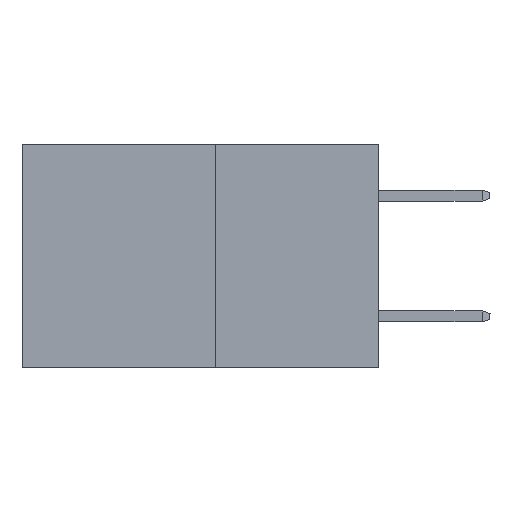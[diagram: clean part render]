
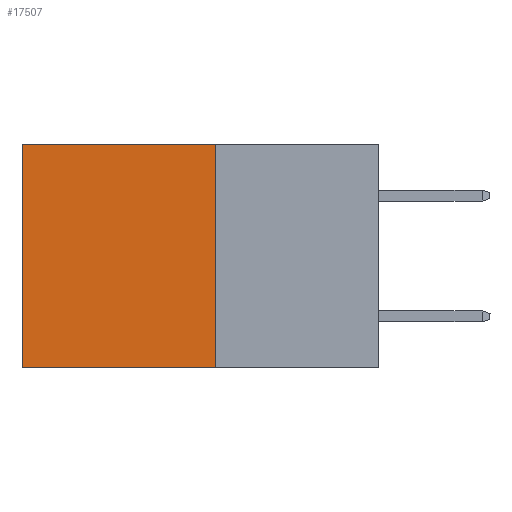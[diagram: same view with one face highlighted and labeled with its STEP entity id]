
A CAD part, left-side view. The second image highlights one B-rep face of the part: STEP entity #17507.
In plain terms, the highlighted planar face has unit normal (-1, 0, 0).
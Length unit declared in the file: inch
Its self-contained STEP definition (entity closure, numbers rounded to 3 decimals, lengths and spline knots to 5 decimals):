
#2429 = LINE ( 'NONE', #11692, #23320 ) ;
#3173 = EDGE_CURVE ( 'NONE', #24598, #13767, #14468, .T. ) ;
#4487 = VERTEX_POINT ( 'NONE', #9803 ) ;
#5060 = AXIS2_PLACEMENT_3D ( 'NONE', #27791, #23147, #8658 ) ;
#5334 = VERTEX_POINT ( 'NONE', #18171 ) ;
#6518 = EDGE_CURVE ( 'NONE', #4487, #5334, #2429, .T. ) ;
#7729 = CARTESIAN_POINT ( 'NONE',  ( 0.277, 0.27, -0.37 ) ) ;
#7737 = ORIENTED_EDGE ( 'NONE', *, *, #30972, .T. ) ;
#8658 = DIRECTION ( 'NONE',  ( 0., 0., -1. ) ) ;
#9319 = ORIENTED_EDGE ( 'NONE', *, *, #6518, .F. ) ;
#9803 = CARTESIAN_POINT ( 'NONE',  ( 0.277, 0.27, 0. ) ) ;
#10033 = FACE_OUTER_BOUND ( 'NONE', #12691, .T. ) ;
#10631 = EDGE_CURVE ( 'NONE', #5334, #13767, #21751, .T. ) ;
#10875 = VECTOR ( 'NONE', #20563, 39.37008 ) ;
#11692 = CARTESIAN_POINT ( 'NONE',  ( 0.277, 0.27, -0.37 ) ) ;
#12691 = EDGE_LOOP ( 'NONE', ( #21202, #16113, #9319, #7737 ) ) ;
#13726 = VECTOR ( 'NONE', #25982, 39.37008 ) ;
#13767 = VERTEX_POINT ( 'NONE', #25356 ) ;
#14468 = LINE ( 'NONE', #25366, #13726 ) ;
#15252 = CARTESIAN_POINT ( 'NONE',  ( 0.277, 0.59, 0. ) ) ;
#16113 = ORIENTED_EDGE ( 'NONE', *, *, #10631, .F. ) ;
#17353 = LINE ( 'NONE', #22896, #10875 ) ;
#17507 = ADVANCED_FACE ( 'NONE', ( #10033 ), #20708, .F. ) ;
#18171 = CARTESIAN_POINT ( 'NONE',  ( 0.277, 0.27, -0.37 ) ) ;
#20563 = DIRECTION ( 'NONE',  ( 0., 1., 0. ) ) ;
#20708 = PLANE ( 'NONE',  #5060 ) ;
#20998 = VECTOR ( 'NONE', #29422, 39.37008 ) ;
#21202 = ORIENTED_EDGE ( 'NONE', *, *, #3173, .T. ) ;
#21751 = LINE ( 'NONE', #7729, #20998 ) ;
#22896 = CARTESIAN_POINT ( 'NONE',  ( 0.277, 0.27, 0. ) ) ;
#23147 = DIRECTION ( 'NONE',  ( 1., 0., 0. ) ) ;
#23320 = VECTOR ( 'NONE', #28483, 39.37008 ) ;
#24598 = VERTEX_POINT ( 'NONE', #15252 ) ;
#25356 = CARTESIAN_POINT ( 'NONE',  ( 0.277, 0.59, -0.37 ) ) ;
#25366 = CARTESIAN_POINT ( 'NONE',  ( 0.277, 0.59, -0.37 ) ) ;
#25982 = DIRECTION ( 'NONE',  ( 0., 0., -1. ) ) ;
#27791 = CARTESIAN_POINT ( 'NONE',  ( 0.277, 0.27, -0.37 ) ) ;
#28483 = DIRECTION ( 'NONE',  ( 0., 0., -1. ) ) ;
#29422 = DIRECTION ( 'NONE',  ( 0., 1., 0. ) ) ;
#30972 = EDGE_CURVE ( 'NONE', #4487, #24598, #17353, .T. ) ;
